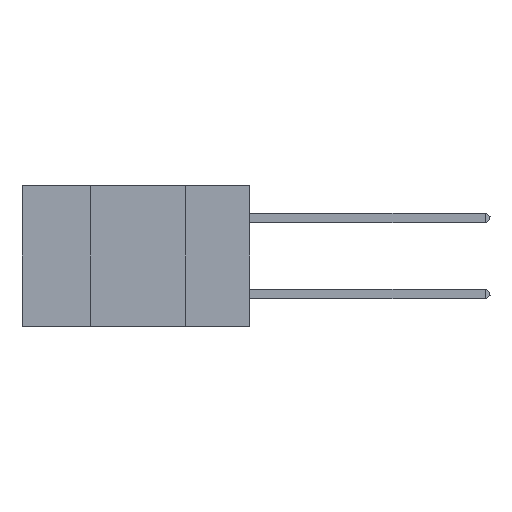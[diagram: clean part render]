
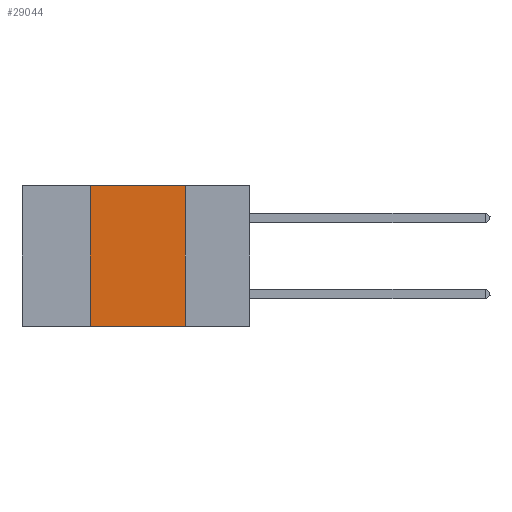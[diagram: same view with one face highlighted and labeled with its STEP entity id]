
A CAD part, left-side view. The second image highlights one B-rep face of the part: STEP entity #29044.
In plain terms, the highlighted planar face has unit normal (-1, 0, 0).
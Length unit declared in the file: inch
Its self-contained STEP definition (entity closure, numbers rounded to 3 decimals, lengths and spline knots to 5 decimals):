
#673 = DIRECTION ( 'NONE',  ( 0., -1., 0. ) ) ;
#1554 = VECTOR ( 'NONE', #673, 39.37008 ) ;
#1571 = LINE ( 'NONE', #10424, #14526 ) ;
#1984 = CARTESIAN_POINT ( 'NONE',  ( 0., 0.17, -0.37 ) ) ;
#3150 = ORIENTED_EDGE ( 'NONE', *, *, #19375, .T. ) ;
#4757 = VECTOR ( 'NONE', #12996, 39.37008 ) ;
#6470 = ORIENTED_EDGE ( 'NONE', *, *, #22298, .F. ) ;
#8403 = FACE_OUTER_BOUND ( 'NONE', #31967, .T. ) ;
#8895 = VERTEX_POINT ( 'NONE', #13791 ) ;
#9765 = LINE ( 'NONE', #33100, #1554 ) ;
#10015 = ORIENTED_EDGE ( 'NONE', *, *, #27286, .F. ) ;
#10424 = CARTESIAN_POINT ( 'NONE',  ( 0., 0.6, -0.37 ) ) ;
#11322 = DIRECTION ( 'NONE',  ( 0., 0., -1. ) ) ;
#12996 = DIRECTION ( 'NONE',  ( 0., 0., 1. ) ) ;
#13791 = CARTESIAN_POINT ( 'NONE',  ( 0., 0.17, 0. ) ) ;
#13868 = AXIS2_PLACEMENT_3D ( 'NONE', #27122, #16599, #24696 ) ;
#14526 = VECTOR ( 'NONE', #29238, 39.37008 ) ;
#16599 = DIRECTION ( 'NONE',  ( 1., 0., 0. ) ) ;
#17685 = CARTESIAN_POINT ( 'NONE',  ( 0., 0.42, 0. ) ) ;
#19227 = VERTEX_POINT ( 'NONE', #26071 ) ;
#19355 = VERTEX_POINT ( 'NONE', #1984 ) ;
#19375 = EDGE_CURVE ( 'NONE', #19227, #19355, #1571, .T. ) ;
#19385 = LINE ( 'NONE', #29067, #4757 ) ;
#22298 = EDGE_CURVE ( 'NONE', #8895, #19355, #22536, .T. ) ;
#22536 = LINE ( 'NONE', #27460, #27818 ) ;
#24696 = DIRECTION ( 'NONE',  ( 0., 0., -1. ) ) ;
#26071 = CARTESIAN_POINT ( 'NONE',  ( 0., 0.42, -0.37 ) ) ;
#27122 = CARTESIAN_POINT ( 'NONE',  ( 0., 0.6, 0. ) ) ;
#27286 = EDGE_CURVE ( 'NONE', #31441, #8895, #9765, .T. ) ;
#27460 = CARTESIAN_POINT ( 'NONE',  ( 0., 0.17, 0. ) ) ;
#27818 = VECTOR ( 'NONE', #11322, 39.37008 ) ;
#29044 = ADVANCED_FACE ( 'NONE', ( #8403 ), #29768, .F. ) ;
#29067 = CARTESIAN_POINT ( 'NONE',  ( 0., 0.42, 0. ) ) ;
#29238 = DIRECTION ( 'NONE',  ( 0., -1., 0. ) ) ;
#29388 = ORIENTED_EDGE ( 'NONE', *, *, #31669, .F. ) ;
#29768 = PLANE ( 'NONE',  #13868 ) ;
#31441 = VERTEX_POINT ( 'NONE', #17685 ) ;
#31669 = EDGE_CURVE ( 'NONE', #19227, #31441, #19385, .T. ) ;
#31967 = EDGE_LOOP ( 'NONE', ( #6470, #10015, #29388, #3150 ) ) ;
#33100 = CARTESIAN_POINT ( 'NONE',  ( 0., 0.6, 0. ) ) ;
